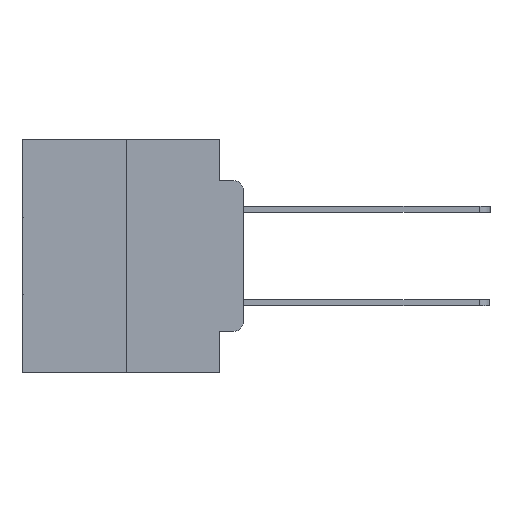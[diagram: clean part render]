
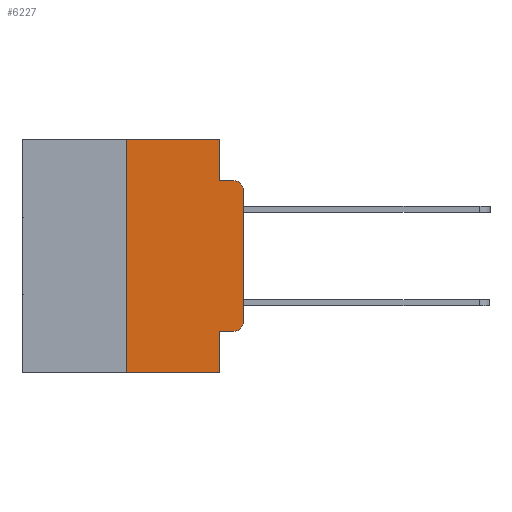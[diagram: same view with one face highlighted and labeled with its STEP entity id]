
A CAD part, left-side view. The second image highlights one B-rep face of the part: STEP entity #6227.
In plain terms, the highlighted planar face has unit normal (-1, 0, 0).
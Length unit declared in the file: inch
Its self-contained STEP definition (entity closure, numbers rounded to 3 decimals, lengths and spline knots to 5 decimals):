
#346 = CARTESIAN_POINT ( 'NONE',  ( 0., 0., -0.3915 ) ) ;
#695 = EDGE_CURVE ( 'NONE', #24650, #18897, #10578, .T. ) ;
#1769 = ORIENTED_EDGE ( 'NONE', *, *, #2837, .T. ) ;
#1784 = VERTEX_POINT ( 'NONE', #6616 ) ;
#2239 = EDGE_CURVE ( 'NONE', #7560, #24650, #18203, .T. ) ;
#2837 = EDGE_CURVE ( 'NONE', #1784, #3450, #15358, .T. ) ;
#3003 = CARTESIAN_POINT ( 'NONE',  ( 0., 0.02, -0.0885 ) ) ;
#3438 = CARTESIAN_POINT ( 'NONE',  ( 0., 0.25, 0. ) ) ;
#3450 = VERTEX_POINT ( 'NONE', #14227 ) ;
#3952 = VERTEX_POINT ( 'NONE', #24966 ) ;
#4405 = EDGE_CURVE ( 'NONE', #1784, #12411, #22257, .T. ) ;
#4916 = AXIS2_PLACEMENT_3D ( 'NONE', #7596, #23304, #9888 ) ;
#4934 = VECTOR ( 'NONE', #7954, 39.37008 ) ;
#5086 = ORIENTED_EDGE ( 'NONE', *, *, #695, .T. ) ;
#5642 = DIRECTION ( 'NONE',  ( 0., 0., 1. ) ) ;
#6227 = ADVANCED_FACE ( 'NONE', ( #10626 ), #25871, .F. ) ;
#6568 = CARTESIAN_POINT ( 'NONE',  ( 0., 0.473, -0.5 ) ) ;
#6616 = CARTESIAN_POINT ( 'NONE',  ( 0., 0.051, -0.4115 ) ) ;
#6930 = VERTEX_POINT ( 'NONE', #8209 ) ;
#7560 = VERTEX_POINT ( 'NONE', #346 ) ;
#7596 = CARTESIAN_POINT ( 'NONE',  ( 0., 0.02, -0.3915 ) ) ;
#7626 = ORIENTED_EDGE ( 'NONE', *, *, #2239, .T. ) ;
#7954 = DIRECTION ( 'NONE',  ( 0., 0., -1. ) ) ;
#7958 = CARTESIAN_POINT ( 'NONE',  ( 0., 0.473, 0. ) ) ;
#8209 = CARTESIAN_POINT ( 'NONE',  ( 0., 0.051, 0. ) ) ;
#9888 = DIRECTION ( 'NONE',  ( 0., 0., -1. ) ) ;
#10457 = VERTEX_POINT ( 'NONE', #19285 ) ;
#10578 = CIRCLE ( 'NONE', #20619, 0.02 ) ;
#10626 = FACE_OUTER_BOUND ( 'NONE', #11119, .T. ) ;
#11027 = CARTESIAN_POINT ( 'NONE',  ( 0., 0.051, -0.0885 ) ) ;
#11119 = EDGE_LOOP ( 'NONE', ( #7626, #5086, #17865, #27946, #16841, #22755, #28903, #17829, #1769, #20640 ) ) ;
#11355 = EDGE_CURVE ( 'NONE', #10457, #12411, #24523, .T. ) ;
#11716 = DIRECTION ( 'NONE',  ( -1., 0., 0. ) ) ;
#11978 = CARTESIAN_POINT ( 'NONE',  ( 0., 0.051, -0.0885 ) ) ;
#12092 = DIRECTION ( 'NONE',  ( 0., 0., -1. ) ) ;
#12212 = VECTOR ( 'NONE', #14207, 39.37008 ) ;
#12219 = DIRECTION ( 'NONE',  ( 0., -1., 0. ) ) ;
#12411 = VERTEX_POINT ( 'NONE', #19868 ) ;
#12600 = CARTESIAN_POINT ( 'NONE',  ( 0., 0.051, 0. ) ) ;
#12634 = VECTOR ( 'NONE', #28974, 39.37008 ) ;
#12849 = LINE ( 'NONE', #3438, #18148 ) ;
#13511 = VECTOR ( 'NONE', #26615, 39.37008 ) ;
#13843 = VECTOR ( 'NONE', #12219, 39.37008 ) ;
#14207 = DIRECTION ( 'NONE',  ( 0., 0., 1. ) ) ;
#14227 = CARTESIAN_POINT ( 'NONE',  ( 0., 0.02, -0.4115 ) ) ;
#14673 = DIRECTION ( 'NONE',  ( 1., 0., 0. ) ) ;
#15328 = VERTEX_POINT ( 'NONE', #11978 ) ;
#15358 = LINE ( 'NONE', #22572, #26480 ) ;
#16604 = EDGE_CURVE ( 'NONE', #10457, #3952, #12849, .T. ) ;
#16841 = ORIENTED_EDGE ( 'NONE', *, *, #17194, .F. ) ;
#16903 = CARTESIAN_POINT ( 'NONE',  ( 0., 0.051, 0. ) ) ;
#17194 = EDGE_CURVE ( 'NONE', #3952, #6930, #19854, .T. ) ;
#17294 = LINE ( 'NONE', #16903, #28379 ) ;
#17658 = CARTESIAN_POINT ( 'NONE',  ( 0., 0., 0. ) ) ;
#17829 = ORIENTED_EDGE ( 'NONE', *, *, #4405, .F. ) ;
#17865 = ORIENTED_EDGE ( 'NONE', *, *, #21101, .F. ) ;
#18148 = VECTOR ( 'NONE', #5642, 39.37008 ) ;
#18203 = LINE ( 'NONE', #17658, #12212 ) ;
#18897 = VERTEX_POINT ( 'NONE', #3003 ) ;
#19164 = DIRECTION ( 'NONE',  ( 0., 0., -1. ) ) ;
#19285 = CARTESIAN_POINT ( 'NONE',  ( 0., 0.25, -0.5 ) ) ;
#19598 = EDGE_CURVE ( 'NONE', #6930, #15328, #17294, .T. ) ;
#19854 = LINE ( 'NONE', #23483, #13843 ) ;
#19868 = CARTESIAN_POINT ( 'NONE',  ( 0., 0.051, -0.5 ) ) ;
#20045 = DIRECTION ( 'NONE',  ( 0., -1., 0. ) ) ;
#20152 = EDGE_CURVE ( 'NONE', #3450, #7560, #20417, .T. ) ;
#20417 = CIRCLE ( 'NONE', #4916, 0.02 ) ;
#20619 = AXIS2_PLACEMENT_3D ( 'NONE', #28555, #11716, #12092 ) ;
#20640 = ORIENTED_EDGE ( 'NONE', *, *, #20152, .T. ) ;
#21101 = EDGE_CURVE ( 'NONE', #15328, #18897, #24724, .T. ) ;
#22257 = LINE ( 'NONE', #12600, #4934 ) ;
#22572 = CARTESIAN_POINT ( 'NONE',  ( 0., 0.051, -0.4115 ) ) ;
#22755 = ORIENTED_EDGE ( 'NONE', *, *, #16604, .F. ) ;
#23304 = DIRECTION ( 'NONE',  ( -1., 0., 0. ) ) ;
#23483 = CARTESIAN_POINT ( 'NONE',  ( 0., 0.473, 0. ) ) ;
#24523 = LINE ( 'NONE', #6568, #12634 ) ;
#24650 = VERTEX_POINT ( 'NONE', #25883 ) ;
#24724 = LINE ( 'NONE', #11027, #13511 ) ;
#24966 = CARTESIAN_POINT ( 'NONE',  ( 0., 0.25, 0. ) ) ;
#25773 = AXIS2_PLACEMENT_3D ( 'NONE', #7958, #14673, #28092 ) ;
#25871 = PLANE ( 'NONE',  #25773 ) ;
#25883 = CARTESIAN_POINT ( 'NONE',  ( 0., 0., -0.1085 ) ) ;
#26480 = VECTOR ( 'NONE', #20045, 39.37008 ) ;
#26615 = DIRECTION ( 'NONE',  ( 0., -1., 0. ) ) ;
#27946 = ORIENTED_EDGE ( 'NONE', *, *, #19598, .F. ) ;
#28092 = DIRECTION ( 'NONE',  ( 0., 0., -1. ) ) ;
#28379 = VECTOR ( 'NONE', #19164, 39.37008 ) ;
#28555 = CARTESIAN_POINT ( 'NONE',  ( 0., 0.02, -0.1085 ) ) ;
#28903 = ORIENTED_EDGE ( 'NONE', *, *, #11355, .T. ) ;
#28974 = DIRECTION ( 'NONE',  ( 0., -1., 0. ) ) ;
